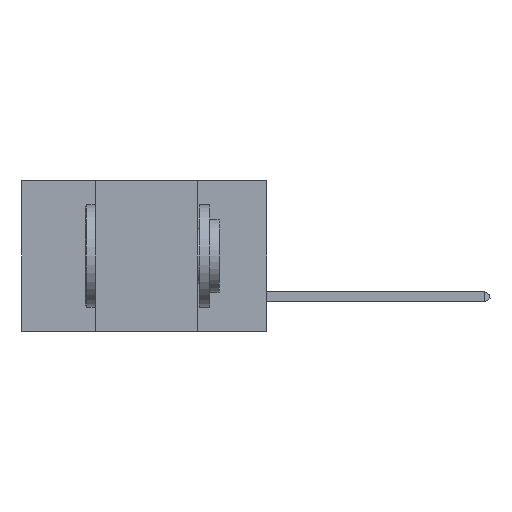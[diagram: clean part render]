
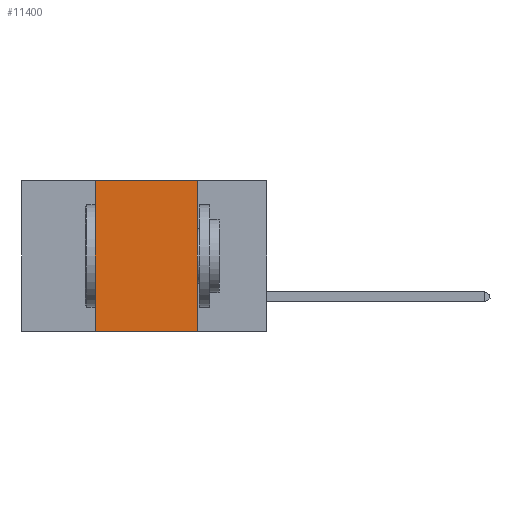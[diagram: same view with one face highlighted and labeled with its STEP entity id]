
A CAD part, left-side view. The second image highlights one B-rep face of the part: STEP entity #11400.
In plain terms, the highlighted planar face has unit normal (-1, 0, 0).
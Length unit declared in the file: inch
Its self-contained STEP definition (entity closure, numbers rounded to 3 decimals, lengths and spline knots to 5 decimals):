
#857 = DIRECTION ( 'NONE',  ( 0., 0., -1. ) ) ;
#2004 = LINE ( 'NONE', #8379, #18442 ) ;
#2569 = CARTESIAN_POINT ( 'NONE',  ( 0., 0.17, -0.37 ) ) ;
#2954 = LINE ( 'NONE', #18194, #11127 ) ;
#3374 = VERTEX_POINT ( 'NONE', #16044 ) ;
#3651 = PLANE ( 'NONE',  #17781 ) ;
#3732 = CARTESIAN_POINT ( 'NONE',  ( 0., 0.6, 0. ) ) ;
#4780 = VECTOR ( 'NONE', #7277, 39.37008 ) ;
#5315 = LINE ( 'NONE', #15131, #4780 ) ;
#5431 = DIRECTION ( 'NONE',  ( 0., 0., -1. ) ) ;
#5472 = EDGE_CURVE ( 'NONE', #17635, #12786, #19844, .T. ) ;
#7094 = ORIENTED_EDGE ( 'NONE', *, *, #11942, .T. ) ;
#7277 = DIRECTION ( 'NONE',  ( 0., -1., 0. ) ) ;
#7582 = CARTESIAN_POINT ( 'NONE',  ( 0., 0.17, 0. ) ) ;
#7651 = CARTESIAN_POINT ( 'NONE',  ( 0., 0.17, 0. ) ) ;
#8067 = EDGE_CURVE ( 'NONE', #3374, #14819, #2954, .T. ) ;
#8379 = CARTESIAN_POINT ( 'NONE',  ( 0., 0.6, -0.37 ) ) ;
#9281 = EDGE_CURVE ( 'NONE', #14819, #17635, #5315, .T. ) ;
#10828 = ORIENTED_EDGE ( 'NONE', *, *, #5472, .F. ) ;
#11127 = VECTOR ( 'NONE', #16699, 39.37008 ) ;
#11244 = VECTOR ( 'NONE', #857, 39.37008 ) ;
#11400 = ADVANCED_FACE ( 'NONE', ( #16128 ), #3651, .F. ) ;
#11942 = EDGE_CURVE ( 'NONE', #3374, #12786, #2004, .T. ) ;
#12786 = VERTEX_POINT ( 'NONE', #2569 ) ;
#13157 = DIRECTION ( 'NONE',  ( 0., -1., 0. ) ) ;
#14819 = VERTEX_POINT ( 'NONE', #20345 ) ;
#14952 = DIRECTION ( 'NONE',  ( 1., 0., 0. ) ) ;
#14993 = ORIENTED_EDGE ( 'NONE', *, *, #9281, .F. ) ;
#15131 = CARTESIAN_POINT ( 'NONE',  ( 0., 0.6, 0. ) ) ;
#16044 = CARTESIAN_POINT ( 'NONE',  ( 0., 0.42, -0.37 ) ) ;
#16128 = FACE_OUTER_BOUND ( 'NONE', #16408, .T. ) ;
#16408 = EDGE_LOOP ( 'NONE', ( #10828, #14993, #18983, #7094 ) ) ;
#16699 = DIRECTION ( 'NONE',  ( 0., 0., 1. ) ) ;
#17635 = VERTEX_POINT ( 'NONE', #7651 ) ;
#17781 = AXIS2_PLACEMENT_3D ( 'NONE', #3732, #14952, #5431 ) ;
#18194 = CARTESIAN_POINT ( 'NONE',  ( 0., 0.42, 0. ) ) ;
#18442 = VECTOR ( 'NONE', #13157, 39.37008 ) ;
#18983 = ORIENTED_EDGE ( 'NONE', *, *, #8067, .F. ) ;
#19844 = LINE ( 'NONE', #7582, #11244 ) ;
#20345 = CARTESIAN_POINT ( 'NONE',  ( 0., 0.42, 0. ) ) ;
